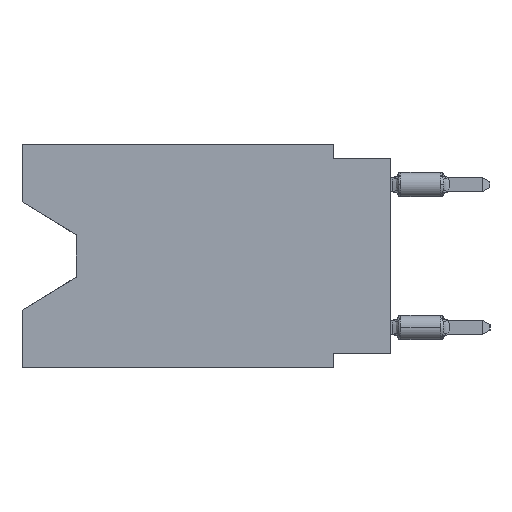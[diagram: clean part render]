
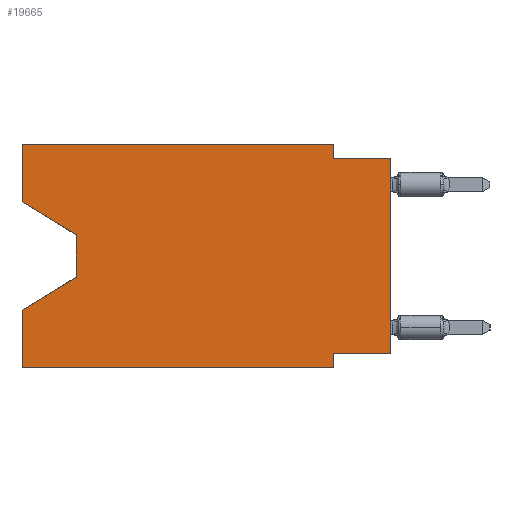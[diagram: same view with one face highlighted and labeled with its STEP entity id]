
A CAD part, left-side view. The second image highlights one B-rep face of the part: STEP entity #19665.
In plain terms, the highlighted planar face has unit normal (-1, 0, 0).
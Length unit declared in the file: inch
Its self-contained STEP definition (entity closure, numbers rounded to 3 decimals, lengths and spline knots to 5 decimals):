
#238 = VECTOR ( 'NONE', #7086, 39.37008 ) ;
#501 = ORIENTED_EDGE ( 'NONE', *, *, #18702, .T. ) ;
#730 = DIRECTION ( 'NONE',  ( 0., 0., -1. ) ) ;
#788 = CARTESIAN_POINT ( 'NONE',  ( 0., 0., -0.365 ) ) ;
#828 = VERTEX_POINT ( 'NONE', #23003 ) ;
#1026 = VERTEX_POINT ( 'NONE', #7272 ) ;
#1476 = DIRECTION ( 'NONE',  ( 0., 0., 1. ) ) ;
#2013 = EDGE_CURVE ( 'NONE', #15789, #19843, #17073, .T. ) ;
#2143 = FACE_OUTER_BOUND ( 'NONE', #32340, .T. ) ;
#2723 = EDGE_CURVE ( 'NONE', #21053, #2958, #29954, .T. ) ;
#2953 = VECTOR ( 'NONE', #14645, 39.37008 ) ;
#2958 = VERTEX_POINT ( 'NONE', #31420 ) ;
#3279 = DIRECTION ( 'NONE',  ( 0., 0., 1. ) ) ;
#3512 = VECTOR ( 'NONE', #28851, 39.37008 ) ;
#4552 = CARTESIAN_POINT ( 'NONE',  ( 0., 0.645, -0.10025 ) ) ;
#4595 = CARTESIAN_POINT ( 'NONE',  ( 0., 0.1, 0. ) ) ;
#4921 = LINE ( 'NONE', #4595, #16059 ) ;
#5127 = EDGE_CURVE ( 'NONE', #27796, #14803, #18531, .T. ) ;
#5542 = EDGE_CURVE ( 'NONE', #828, #2958, #20991, .T. ) ;
#6374 = LINE ( 'NONE', #28782, #15822 ) ;
#7086 = DIRECTION ( 'NONE',  ( 0., -1., 0. ) ) ;
#7229 = EDGE_CURVE ( 'NONE', #13979, #21053, #23428, .T. ) ;
#7249 = LINE ( 'NONE', #27304, #238 ) ;
#7272 = CARTESIAN_POINT ( 'NONE',  ( 0., 0.1, 0. ) ) ;
#7368 = CARTESIAN_POINT ( 'NONE',  ( 0., 0.645, 0. ) ) ;
#7391 = CARTESIAN_POINT ( 'NONE',  ( 0., 0.55, -0.232 ) ) ;
#8256 = LINE ( 'NONE', #788, #22808 ) ;
#8501 = ORIENTED_EDGE ( 'NONE', *, *, #17276, .F. ) ;
#8677 = CARTESIAN_POINT ( 'NONE',  ( 0., 0.55, -0.158 ) ) ;
#9141 = ORIENTED_EDGE ( 'NONE', *, *, #16417, .T. ) ;
#9165 = VECTOR ( 'NONE', #22364, 39.37008 ) ;
#9339 = VECTOR ( 'NONE', #3279, 39.37008 ) ;
#9774 = CARTESIAN_POINT ( 'NONE',  ( 0., 0.645, 0. ) ) ;
#10577 = CARTESIAN_POINT ( 'NONE',  ( 0., 0.645, -0.10025 ) ) ;
#11263 = CARTESIAN_POINT ( 'NONE',  ( 0., 0., 0. ) ) ;
#12253 = PLANE ( 'NONE',  #31000 ) ;
#12387 = ORIENTED_EDGE ( 'NONE', *, *, #18238, .T. ) ;
#13979 = VERTEX_POINT ( 'NONE', #32656 ) ;
#14013 = ORIENTED_EDGE ( 'NONE', *, *, #30738, .F. ) ;
#14095 = VERTEX_POINT ( 'NONE', #31149 ) ;
#14212 = VERTEX_POINT ( 'NONE', #19168 ) ;
#14645 = DIRECTION ( 'NONE',  ( 0., -0.855, -0.519 ) ) ;
#14803 = VERTEX_POINT ( 'NONE', #7368 ) ;
#15503 = VECTOR ( 'NONE', #17873, 39.37008 ) ;
#15789 = VERTEX_POINT ( 'NONE', #16165 ) ;
#15822 = VECTOR ( 'NONE', #18790, 39.37008 ) ;
#15860 = VECTOR ( 'NONE', #1476, 39.37008 ) ;
#16059 = VECTOR ( 'NONE', #17166, 39.37008 ) ;
#16165 = CARTESIAN_POINT ( 'NONE',  ( 0., 0.1, -0.025 ) ) ;
#16417 = EDGE_CURVE ( 'NONE', #26973, #19843, #29026, .T. ) ;
#17073 = LINE ( 'NONE', #27201, #9165 ) ;
#17108 = ORIENTED_EDGE ( 'NONE', *, *, #2013, .F. ) ;
#17166 = DIRECTION ( 'NONE',  ( 0., 0., -1. ) ) ;
#17276 = EDGE_CURVE ( 'NONE', #14212, #14095, #6374, .T. ) ;
#17593 = ORIENTED_EDGE ( 'NONE', *, *, #2723, .T. ) ;
#17873 = DIRECTION ( 'NONE',  ( 0., -1., 0. ) ) ;
#18238 = EDGE_CURVE ( 'NONE', #828, #14095, #7249, .T. ) ;
#18248 = EDGE_CURVE ( 'NONE', #1026, #15789, #4921, .T. ) ;
#18351 = DIRECTION ( 'NONE',  ( 0., 1., 0. ) ) ;
#18531 = LINE ( 'NONE', #29176, #3512 ) ;
#18702 = EDGE_CURVE ( 'NONE', #27796, #13979, #19614, .T. ) ;
#18790 = DIRECTION ( 'NONE',  ( 0., 0., -1. ) ) ;
#19168 = CARTESIAN_POINT ( 'NONE',  ( 0., 0.1, -0.365 ) ) ;
#19614 = LINE ( 'NONE', #4552, #2953 ) ;
#19665 = ADVANCED_FACE ( 'NONE', ( #2143 ), #12253, .F. ) ;
#19843 = VERTEX_POINT ( 'NONE', #22262 ) ;
#19875 = DIRECTION ( 'NONE',  ( 0., 0., -1. ) ) ;
#20693 = LINE ( 'NONE', #30668, #15503 ) ;
#20991 = LINE ( 'NONE', #31132, #9339 ) ;
#21053 = VERTEX_POINT ( 'NONE', #7391 ) ;
#21374 = VECTOR ( 'NONE', #22279, 39.37008 ) ;
#22262 = CARTESIAN_POINT ( 'NONE',  ( 0., 0., -0.025 ) ) ;
#22279 = DIRECTION ( 'NONE',  ( 0., 0.855, -0.519 ) ) ;
#22364 = DIRECTION ( 'NONE',  ( 0., -1., 0. ) ) ;
#22446 = CARTESIAN_POINT ( 'NONE',  ( 0., 0.55, -0.232 ) ) ;
#22808 = VECTOR ( 'NONE', #18351, 39.37008 ) ;
#22824 = ORIENTED_EDGE ( 'NONE', *, *, #7229, .T. ) ;
#23003 = CARTESIAN_POINT ( 'NONE',  ( 0., 0.645, -0.39 ) ) ;
#23428 = LINE ( 'NONE', #8677, #31081 ) ;
#24473 = ORIENTED_EDGE ( 'NONE', *, *, #5127, .F. ) ;
#26973 = VERTEX_POINT ( 'NONE', #28430 ) ;
#27201 = CARTESIAN_POINT ( 'NONE',  ( 0., 0., -0.025 ) ) ;
#27304 = CARTESIAN_POINT ( 'NONE',  ( 0., 0.645, -0.39 ) ) ;
#27519 = DIRECTION ( 'NONE',  ( 1., 0., 0. ) ) ;
#27796 = VERTEX_POINT ( 'NONE', #10577 ) ;
#28312 = ORIENTED_EDGE ( 'NONE', *, *, #29105, .F. ) ;
#28430 = CARTESIAN_POINT ( 'NONE',  ( 0., 0., -0.365 ) ) ;
#28782 = CARTESIAN_POINT ( 'NONE',  ( 0., 0.1, -0.39 ) ) ;
#28851 = DIRECTION ( 'NONE',  ( 0., 0., 1. ) ) ;
#29026 = LINE ( 'NONE', #11263, #15860 ) ;
#29105 = EDGE_CURVE ( 'NONE', #26973, #14212, #8256, .T. ) ;
#29176 = CARTESIAN_POINT ( 'NONE',  ( 0., 0.645, 0. ) ) ;
#29214 = ORIENTED_EDGE ( 'NONE', *, *, #5542, .F. ) ;
#29954 = LINE ( 'NONE', #22446, #21374 ) ;
#30668 = CARTESIAN_POINT ( 'NONE',  ( 0., 0.645, 0. ) ) ;
#30738 = EDGE_CURVE ( 'NONE', #14803, #1026, #20693, .T. ) ;
#31000 = AXIS2_PLACEMENT_3D ( 'NONE', #9774, #27519, #19875 ) ;
#31081 = VECTOR ( 'NONE', #730, 39.37008 ) ;
#31132 = CARTESIAN_POINT ( 'NONE',  ( 0., 0.645, 0. ) ) ;
#31149 = CARTESIAN_POINT ( 'NONE',  ( 0., 0.1, -0.39 ) ) ;
#31288 = ORIENTED_EDGE ( 'NONE', *, *, #18248, .F. ) ;
#31420 = CARTESIAN_POINT ( 'NONE',  ( 0., 0.645, -0.28975 ) ) ;
#32340 = EDGE_LOOP ( 'NONE', ( #501, #22824, #17593, #29214, #12387, #8501, #28312, #9141, #17108, #31288, #14013, #24473 ) ) ;
#32656 = CARTESIAN_POINT ( 'NONE',  ( 0., 0.55, -0.158 ) ) ;
